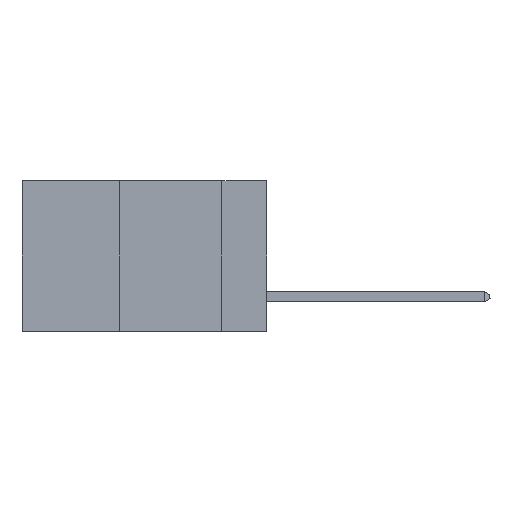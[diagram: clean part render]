
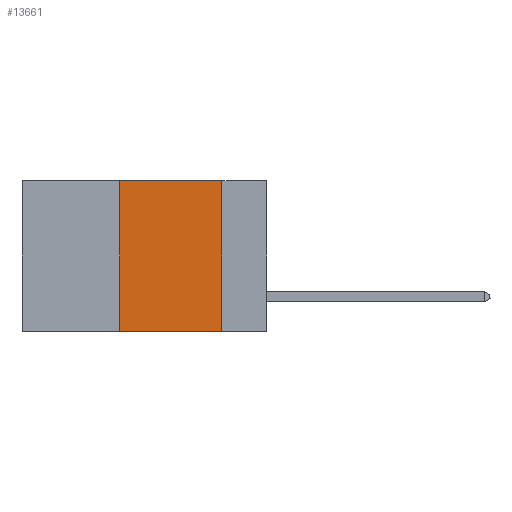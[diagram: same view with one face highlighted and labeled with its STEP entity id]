
A CAD part, left-side view. The second image highlights one B-rep face of the part: STEP entity #13661.
In plain terms, the highlighted planar face has unit normal (-1, 0, 0).
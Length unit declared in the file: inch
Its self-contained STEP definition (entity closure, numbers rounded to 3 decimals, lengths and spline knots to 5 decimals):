
#721 = CARTESIAN_POINT ( 'NONE',  ( 0., 0.36, 0. ) ) ;
#1833 = VERTEX_POINT ( 'NONE', #33689 ) ;
#2607 = DIRECTION ( 'NONE',  ( 1., 0., 0. ) ) ;
#3160 = LINE ( 'NONE', #34993, #14258 ) ;
#3231 = CARTESIAN_POINT ( 'NONE',  ( 0., 0.36, -0.37 ) ) ;
#4096 = VECTOR ( 'NONE', #35812, 39.37008 ) ;
#7024 = CARTESIAN_POINT ( 'NONE',  ( 0., 0.36, 0. ) ) ;
#8995 = FACE_OUTER_BOUND ( 'NONE', #27728, .T. ) ;
#9282 = ORIENTED_EDGE ( 'NONE', *, *, #15409, .T. ) ;
#9540 = DIRECTION ( 'NONE',  ( 0., -1., 0. ) ) ;
#10803 = CARTESIAN_POINT ( 'NONE',  ( 0., 0.11, 0. ) ) ;
#11138 = EDGE_CURVE ( 'NONE', #26168, #38061, #3160, .T. ) ;
#13661 = ADVANCED_FACE ( 'NONE', ( #8995 ), #16869, .F. ) ;
#14258 = VECTOR ( 'NONE', #9540, 39.37008 ) ;
#15409 = EDGE_CURVE ( 'NONE', #20242, #1833, #35612, .T. ) ;
#15596 = LINE ( 'NONE', #721, #28907 ) ;
#15870 = ORIENTED_EDGE ( 'NONE', *, *, #37790, .F. ) ;
#16735 = VECTOR ( 'NONE', #26020, 39.37008 ) ;
#16869 = PLANE ( 'NONE',  #21961 ) ;
#20242 = VERTEX_POINT ( 'NONE', #3231 ) ;
#21961 = AXIS2_PLACEMENT_3D ( 'NONE', #38294, #2607, #34876 ) ;
#22284 = DIRECTION ( 'NONE',  ( 0., 0., 1. ) ) ;
#26020 = DIRECTION ( 'NONE',  ( 0., -1., 0. ) ) ;
#26168 = VERTEX_POINT ( 'NONE', #7024 ) ;
#26538 = ORIENTED_EDGE ( 'NONE', *, *, #43178, .F. ) ;
#27728 = EDGE_LOOP ( 'NONE', ( #15870, #36506, #26538, #9282 ) ) ;
#28715 = CARTESIAN_POINT ( 'NONE',  ( 0., 0.11, 0. ) ) ;
#28907 = VECTOR ( 'NONE', #22284, 39.37008 ) ;
#33689 = CARTESIAN_POINT ( 'NONE',  ( 0., 0.11, -0.37 ) ) ;
#34876 = DIRECTION ( 'NONE',  ( 0., 0., -1. ) ) ;
#34993 = CARTESIAN_POINT ( 'NONE',  ( 0., 0.6, 0. ) ) ;
#35612 = LINE ( 'NONE', #36568, #16735 ) ;
#35812 = DIRECTION ( 'NONE',  ( 0., 0., -1. ) ) ;
#36506 = ORIENTED_EDGE ( 'NONE', *, *, #11138, .F. ) ;
#36568 = CARTESIAN_POINT ( 'NONE',  ( 0., 0.6, -0.37 ) ) ;
#37790 = EDGE_CURVE ( 'NONE', #38061, #1833, #39091, .T. ) ;
#38061 = VERTEX_POINT ( 'NONE', #28715 ) ;
#38294 = CARTESIAN_POINT ( 'NONE',  ( 0., 0.6, 0. ) ) ;
#39091 = LINE ( 'NONE', #10803, #4096 ) ;
#43178 = EDGE_CURVE ( 'NONE', #20242, #26168, #15596, .T. ) ;
